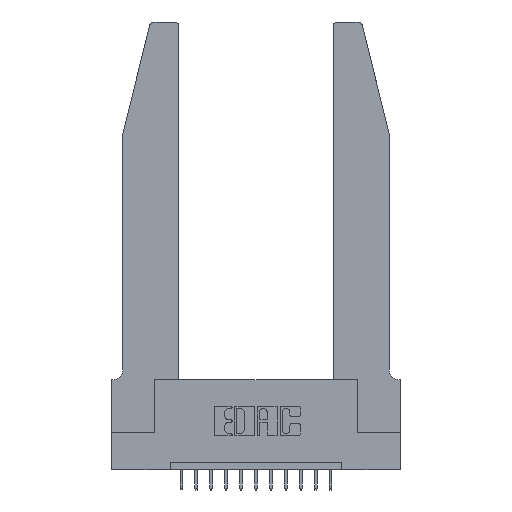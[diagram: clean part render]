
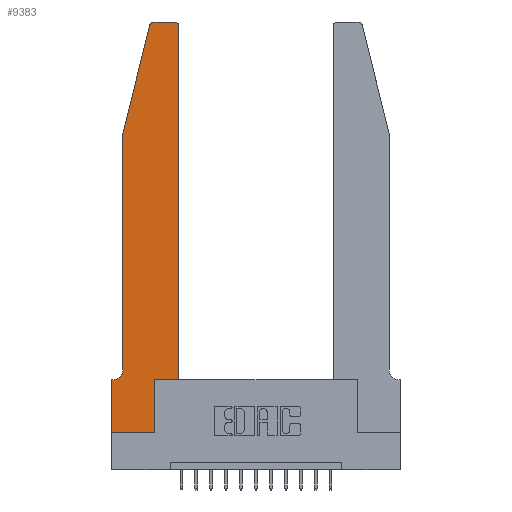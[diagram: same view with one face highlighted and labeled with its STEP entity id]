
A CAD part, top view. The second image highlights one B-rep face of the part: STEP entity #9383.
In plain terms, the highlighted planar face has unit normal (0, 0, 1).
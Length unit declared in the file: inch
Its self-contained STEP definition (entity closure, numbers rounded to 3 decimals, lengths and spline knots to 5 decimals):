
#46 = VERTEX_POINT ( 'NONE', #7421 ) ;
#84 = ORIENTED_EDGE ( 'NONE', *, *, #2708, .T. ) ;
#383 = CARTESIAN_POINT ( 'NONE',  ( 0.0055, 0.35, 0.37 ) ) ;
#574 = ORIENTED_EDGE ( 'NONE', *, *, #13659, .T. ) ;
#819 = VECTOR ( 'NONE', #12088, 39.37008 ) ;
#1027 = EDGE_CURVE ( 'NONE', #4964, #12180, #1107, .T. ) ;
#1086 = ORIENTED_EDGE ( 'NONE', *, *, #13757, .T. ) ;
#1107 = LINE ( 'NONE', #8730, #6194 ) ;
#1415 = VERTEX_POINT ( 'NONE', #383 ) ;
#1617 = CARTESIAN_POINT ( 'NONE',  ( 0.25487, 2.72718, 0.37 ) ) ;
#1831 = VECTOR ( 'NONE', #12895, 39.37008 ) ;
#1886 = CIRCLE ( 'NONE', #14507, 0.03 ) ;
#1887 = VECTOR ( 'NONE', #13596, 39.37008 ) ;
#2525 = CARTESIAN_POINT ( 'NONE',  ( 0.4205, 2.75, 0.37 ) ) ;
#2708 = EDGE_CURVE ( 'NONE', #46, #11713, #11626, .T. ) ;
#2774 = CARTESIAN_POINT ( 'NONE',  ( 0.4505, 0.35, 0.37 ) ) ;
#2781 = EDGE_CURVE ( 'NONE', #7059, #46, #9254, .T. ) ;
#3293 = CARTESIAN_POINT ( 'NONE',  ( 0., 0., 0.37 ) ) ;
#3389 = EDGE_LOOP ( 'NONE', ( #1086, #16754, #10787, #84, #6930, #574, #10072, #9057, #8830, #11661, #7728, #10377 ) ) ;
#3500 = DIRECTION ( 'NONE',  ( -1., 0., 0. ) ) ;
#3537 = DIRECTION ( 'NONE',  ( 0., 0., 1. ) ) ;
#3609 = DIRECTION ( 'NONE',  ( -0.239, -0.971, 0. ) ) ;
#3767 = VECTOR ( 'NONE', #16071, 39.37008 ) ;
#3881 = EDGE_CURVE ( 'NONE', #11713, #1415, #6766, .T. ) ;
#3891 = CARTESIAN_POINT ( 'NONE',  ( 0.2865, 0., 0.37 ) ) ;
#3946 = CARTESIAN_POINT ( 'NONE',  ( 0.0755, 2., 0.37 ) ) ;
#4064 = CARTESIAN_POINT ( 'NONE',  ( 0.0755, 0.35, 0.37 ) ) ;
#4478 = DIRECTION ( 'NONE',  ( 0., 0., 1. ) ) ;
#4821 = LINE ( 'NONE', #14057, #10917 ) ;
#4964 = VERTEX_POINT ( 'NONE', #9846 ) ;
#5535 = VERTEX_POINT ( 'NONE', #2774 ) ;
#5552 = CARTESIAN_POINT ( 'NONE',  ( 0.2865, 0.35, 0.37 ) ) ;
#5572 = VECTOR ( 'NONE', #12709, 39.37008 ) ;
#5708 = LINE ( 'NONE', #15600, #1831 ) ;
#5865 = VERTEX_POINT ( 'NONE', #5552 ) ;
#5887 = DIRECTION ( 'NONE',  ( 1., 0., 0. ) ) ;
#6194 = VECTOR ( 'NONE', #14081, 39.37008 ) ;
#6256 = DIRECTION ( 'NONE',  ( 0., -1., 0. ) ) ;
#6470 = CARTESIAN_POINT ( 'NONE',  ( 0., 0., 0.37 ) ) ;
#6473 = VECTOR ( 'NONE', #3609, 39.37008 ) ;
#6766 = CIRCLE ( 'NONE', #12401, 0.07 ) ;
#6930 = ORIENTED_EDGE ( 'NONE', *, *, #3881, .T. ) ;
#7015 = CARTESIAN_POINT ( 'NONE',  ( 0.2865, 0.35, 0.37 ) ) ;
#7059 = VERTEX_POINT ( 'NONE', #1617 ) ;
#7115 = VERTEX_POINT ( 'NONE', #16349 ) ;
#7421 = CARTESIAN_POINT ( 'NONE',  ( 0.0755, 2., 0.37 ) ) ;
#7599 = DIRECTION ( 'NONE',  ( 0., 0., -1. ) ) ;
#7728 = ORIENTED_EDGE ( 'NONE', *, *, #9295, .T. ) ;
#7850 = CARTESIAN_POINT ( 'NONE',  ( 0.0755, 2., 0.37 ) ) ;
#8014 = CIRCLE ( 'NONE', #8860, 0.03 ) ;
#8247 = LINE ( 'NONE', #7015, #1887 ) ;
#8606 = EDGE_CURVE ( 'NONE', #7115, #16990, #8014, .T. ) ;
#8730 = CARTESIAN_POINT ( 'NONE',  ( 0., 0., 0.37 ) ) ;
#8830 = ORIENTED_EDGE ( 'NONE', *, *, #16642, .T. ) ;
#8842 = AXIS2_PLACEMENT_3D ( 'NONE', #13792, #4478, #5887 ) ;
#8860 = AXIS2_PLACEMENT_3D ( 'NONE', #8919, #3537, #11470 ) ;
#8919 = CARTESIAN_POINT ( 'NONE',  ( 0.4205, 2.72, 0.37 ) ) ;
#9057 = ORIENTED_EDGE ( 'NONE', *, *, #13386, .T. ) ;
#9254 = LINE ( 'NONE', #7850, #6473 ) ;
#9285 = VECTOR ( 'NONE', #6256, 39.37008 ) ;
#9295 = EDGE_CURVE ( 'NONE', #5535, #7115, #14675, .T. ) ;
#9359 = EDGE_CURVE ( 'NONE', #5865, #5535, #5708, .T. ) ;
#9383 = ADVANCED_FACE ( 'NONE', ( #15268 ), #15186, .T. ) ;
#9472 = CARTESIAN_POINT ( 'NONE',  ( 0.284, 2.75, 0.37 ) ) ;
#9775 = CARTESIAN_POINT ( 'NONE',  ( 0.0755, 0.42, 0.37 ) ) ;
#9846 = CARTESIAN_POINT ( 'NONE',  ( 0., 0.35, 0.37 ) ) ;
#9966 = CARTESIAN_POINT ( 'NONE',  ( 0.0055, 0.42, 0.37 ) ) ;
#10072 = ORIENTED_EDGE ( 'NONE', *, *, #1027, .T. ) ;
#10377 = ORIENTED_EDGE ( 'NONE', *, *, #8606, .T. ) ;
#10787 = ORIENTED_EDGE ( 'NONE', *, *, #2781, .T. ) ;
#10917 = VECTOR ( 'NONE', #3500, 39.37008 ) ;
#11356 = EDGE_CURVE ( 'NONE', #14378, #7059, #1886, .T. ) ;
#11470 = DIRECTION ( 'NONE',  ( 1., 0., 0. ) ) ;
#11626 = LINE ( 'NONE', #3946, #9285 ) ;
#11661 = ORIENTED_EDGE ( 'NONE', *, *, #9359, .T. ) ;
#11713 = VERTEX_POINT ( 'NONE', #9775 ) ;
#12088 = DIRECTION ( 'NONE',  ( -1., 0., 0. ) ) ;
#12180 = VERTEX_POINT ( 'NONE', #6470 ) ;
#12259 = LINE ( 'NONE', #4064, #819 ) ;
#12401 = AXIS2_PLACEMENT_3D ( 'NONE', #9966, #7599, #15301 ) ;
#12612 = DIRECTION ( 'NONE',  ( 1., 0., 0. ) ) ;
#12709 = DIRECTION ( 'NONE',  ( 1., 0., 0. ) ) ;
#12895 = DIRECTION ( 'NONE',  ( 1., 0., 0. ) ) ;
#13386 = EDGE_CURVE ( 'NONE', #12180, #15951, #15325, .T. ) ;
#13596 = DIRECTION ( 'NONE',  ( 0., 1., 0. ) ) ;
#13659 = EDGE_CURVE ( 'NONE', #1415, #4964, #12259, .T. ) ;
#13757 = EDGE_CURVE ( 'NONE', #16990, #14378, #4821, .T. ) ;
#13792 = CARTESIAN_POINT ( 'NONE',  ( 0., 0.35, 0.37 ) ) ;
#14057 = CARTESIAN_POINT ( 'NONE',  ( 0.2605, 2.75, 0.37 ) ) ;
#14081 = DIRECTION ( 'NONE',  ( 0., -1., 0. ) ) ;
#14378 = VERTEX_POINT ( 'NONE', #9472 ) ;
#14507 = AXIS2_PLACEMENT_3D ( 'NONE', #16869, #15647, #12612 ) ;
#14675 = LINE ( 'NONE', #16329, #3767 ) ;
#15186 = PLANE ( 'NONE',  #8842 ) ;
#15268 = FACE_OUTER_BOUND ( 'NONE', #3389, .T. ) ;
#15301 = DIRECTION ( 'NONE',  ( -1., 0., 0. ) ) ;
#15325 = LINE ( 'NONE', #3293, #5572 ) ;
#15600 = CARTESIAN_POINT ( 'NONE',  ( 0.4505, 0.35, 0.37 ) ) ;
#15647 = DIRECTION ( 'NONE',  ( 0., 0., 1. ) ) ;
#15951 = VERTEX_POINT ( 'NONE', #3891 ) ;
#16071 = DIRECTION ( 'NONE',  ( 0., 1., 0. ) ) ;
#16329 = CARTESIAN_POINT ( 'NONE',  ( 0.4505, 0.35, 0.37 ) ) ;
#16349 = CARTESIAN_POINT ( 'NONE',  ( 0.4505, 2.72, 0.37 ) ) ;
#16642 = EDGE_CURVE ( 'NONE', #15951, #5865, #8247, .T. ) ;
#16754 = ORIENTED_EDGE ( 'NONE', *, *, #11356, .T. ) ;
#16869 = CARTESIAN_POINT ( 'NONE',  ( 0.284, 2.72, 0.37 ) ) ;
#16990 = VERTEX_POINT ( 'NONE', #2525 ) ;
